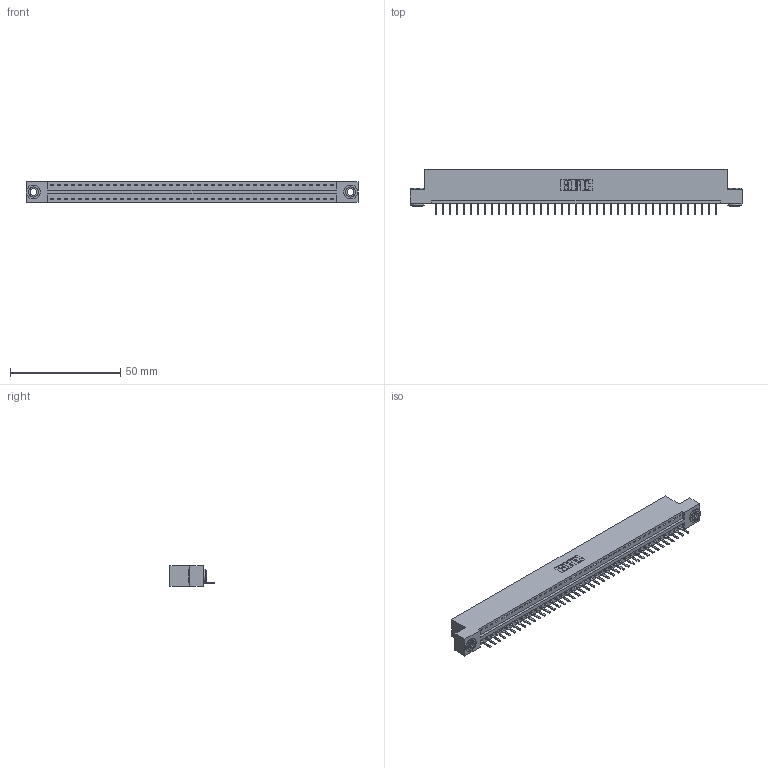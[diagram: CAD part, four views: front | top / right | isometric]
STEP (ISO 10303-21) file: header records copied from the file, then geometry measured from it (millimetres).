
FILE_DESCRIPTION (( 'STEP AP203' ), '1' );
FILE_NAME ('396-041-520-103.STEP', '2018-09-06T22:11:18', ( '' ), ( '' ), 'SwSTEP 2.0', 'SolidWorks 2016', '' );
FILE_SCHEMA (( 'CONFIG_CONTROL_DESIGN' ));
Length unit declared in the file: inch
Products named in the file (4): 345-292-001_345-293-120; 345-250-002_345-250-002-102; 396-041-520-103; 346 Part_Flush Mounting Lugs - 0.156 Dia-TH
Assembly tree (44 placements, depth 2):
  396-041-520-103
    346 Part_Flush Mounting Lugs - 0.156 Dia-TH
    345-292-001_345-293-120  x41
    345-250-002_345-250-002-102  x2
Bounding box: 150.75 x 20.02 x 9.4 mm (x, y, z)
Volume: 14324.6 mm3; surface area: 17718.6 mm2
Topology: 44 solids, 44 shells, 2702 faces, 7949 edges, 5186 vertices
Faces by surface type: plane 1808, cylinder 886, cone 8
Entity records: 26344 total; most frequent: CARTESIAN_POINT 4506, ORIENTED_EDGE 4462, DIRECTION 3995, EDGE_CURVE 2231, LINE 1907, VECTOR 1907, VERTEX_POINT 1482, AXIS2_PLACEMENT_3D 1044
